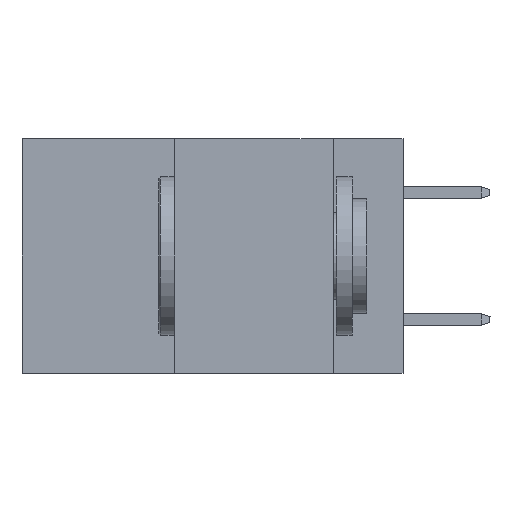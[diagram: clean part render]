
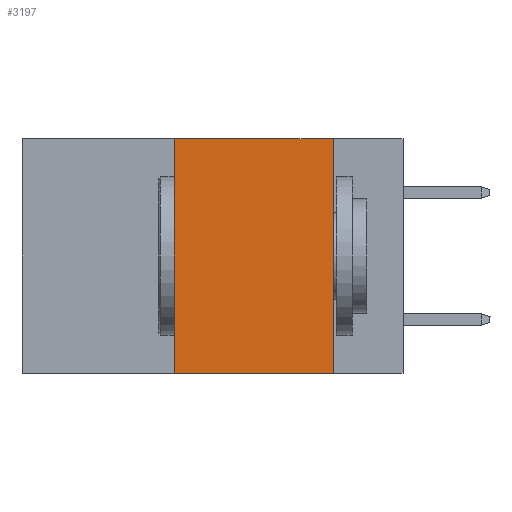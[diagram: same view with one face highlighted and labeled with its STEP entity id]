
A CAD part, left-side view. The second image highlights one B-rep face of the part: STEP entity #3197.
In plain terms, the highlighted planar face has unit normal (-1, 0, 0).
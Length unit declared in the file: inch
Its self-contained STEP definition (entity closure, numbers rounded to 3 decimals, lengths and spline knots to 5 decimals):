
#385 = EDGE_LOOP ( 'NONE', ( #917, #642, #3728, #6059 ) ) ;
#477 = CARTESIAN_POINT ( 'NONE',  ( 0., 0.11, -0.37 ) ) ;
#642 = ORIENTED_EDGE ( 'NONE', *, *, #5744, .F. ) ;
#743 = CARTESIAN_POINT ( 'NONE',  ( 0., 0.11, 0. ) ) ;
#917 = ORIENTED_EDGE ( 'NONE', *, *, #5114, .F. ) ;
#1545 = EDGE_CURVE ( 'NONE', #7890, #9632, #14278, .T. ) ;
#1822 = VECTOR ( 'NONE', #8312, 39.37008 ) ;
#3197 = ADVANCED_FACE ( 'NONE', ( #14961 ), #8943, .F. ) ;
#3621 = LINE ( 'NONE', #10655, #8494 ) ;
#3728 = ORIENTED_EDGE ( 'NONE', *, *, #1545, .F. ) ;
#4149 = VERTEX_POINT ( 'NONE', #477 ) ;
#4255 = DIRECTION ( 'NONE',  ( 0., 0., -1. ) ) ;
#5114 = EDGE_CURVE ( 'NONE', #13983, #4149, #6033, .T. ) ;
#5744 = EDGE_CURVE ( 'NONE', #9632, #13983, #14800, .T. ) ;
#6033 = LINE ( 'NONE', #8389, #1822 ) ;
#6059 = ORIENTED_EDGE ( 'NONE', *, *, #7784, .T. ) ;
#6332 = CARTESIAN_POINT ( 'NONE',  ( 0., 0.6, 0. ) ) ;
#6577 = DIRECTION ( 'NONE',  ( 1., 0., 0. ) ) ;
#7784 = EDGE_CURVE ( 'NONE', #7890, #4149, #3621, .T. ) ;
#7890 = VERTEX_POINT ( 'NONE', #11215 ) ;
#8034 = CARTESIAN_POINT ( 'NONE',  ( 0., 0.36, 0. ) ) ;
#8312 = DIRECTION ( 'NONE',  ( 0., 0., -1. ) ) ;
#8389 = CARTESIAN_POINT ( 'NONE',  ( 0., 0.11, 0. ) ) ;
#8418 = VECTOR ( 'NONE', #14354, 39.37008 ) ;
#8494 = VECTOR ( 'NONE', #11988, 39.37008 ) ;
#8939 = DIRECTION ( 'NONE',  ( 0., -1., 0. ) ) ;
#8943 = PLANE ( 'NONE',  #12228 ) ;
#9632 = VERTEX_POINT ( 'NONE', #8034 ) ;
#10050 = CARTESIAN_POINT ( 'NONE',  ( 0., 0.6, 0. ) ) ;
#10655 = CARTESIAN_POINT ( 'NONE',  ( 0., 0.6, -0.37 ) ) ;
#11215 = CARTESIAN_POINT ( 'NONE',  ( 0., 0.36, -0.37 ) ) ;
#11988 = DIRECTION ( 'NONE',  ( 0., -1., 0. ) ) ;
#12228 = AXIS2_PLACEMENT_3D ( 'NONE', #10050, #6577, #4255 ) ;
#12916 = CARTESIAN_POINT ( 'NONE',  ( 0., 0.36, 0. ) ) ;
#13983 = VERTEX_POINT ( 'NONE', #743 ) ;
#14278 = LINE ( 'NONE', #12916, #8418 ) ;
#14354 = DIRECTION ( 'NONE',  ( 0., 0., 1. ) ) ;
#14800 = LINE ( 'NONE', #6332, #15206 ) ;
#14961 = FACE_OUTER_BOUND ( 'NONE', #385, .T. ) ;
#15206 = VECTOR ( 'NONE', #8939, 39.37008 ) ;
